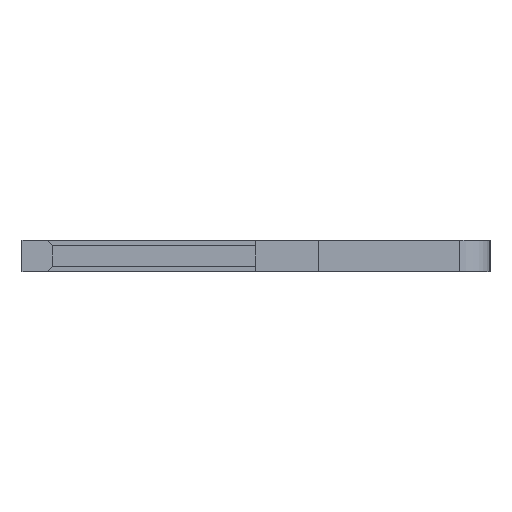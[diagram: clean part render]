
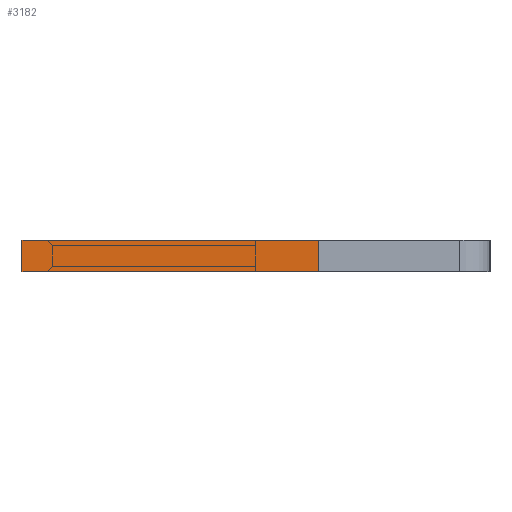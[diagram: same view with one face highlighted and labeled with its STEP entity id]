
A CAD part, left-side view. The second image highlights one B-rep face of the part: STEP entity #3182.
In plain terms, the highlighted face is planar.
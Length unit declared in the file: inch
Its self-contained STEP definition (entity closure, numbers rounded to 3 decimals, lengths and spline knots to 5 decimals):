
#20 = LINE ( 'NONE', #1479, #3089 ) ;
#89 = ORIENTED_EDGE ( 'NONE', *, *, #2340, .T. ) ;
#145 = VERTEX_POINT ( 'NONE', #1949 ) ;
#252 = CARTESIAN_POINT ( 'NONE',  ( 0.01, 0.15, -0.04 ) ) ;
#434 = VECTOR ( 'NONE', #2036, 39.37008 ) ;
#546 = ORIENTED_EDGE ( 'NONE', *, *, #952, .F. ) ;
#728 = CARTESIAN_POINT ( 'NONE',  ( 0.01, -0.04, -0.04 ) ) ;
#780 = DIRECTION ( 'NONE',  ( 0., 1., 0. ) ) ;
#808 = CARTESIAN_POINT ( 'NONE',  ( 0.01, 0.15, -0.04 ) ) ;
#821 = PLANE ( 'NONE',  #4189 ) ;
#865 = EDGE_CURVE ( 'NONE', #3036, #145, #2927, .T. ) ;
#876 = ORIENTED_EDGE ( 'NONE', *, *, #865, .F. ) ;
#952 = EDGE_CURVE ( 'NONE', #4220, #3036, #3999, .T. ) ;
#1039 = ORIENTED_EDGE ( 'NONE', *, *, #2224, .T. ) ;
#1185 = CARTESIAN_POINT ( 'NONE',  ( 0.01, 0.15, -0.04 ) ) ;
#1450 = FACE_OUTER_BOUND ( 'NONE', #3519, .T. ) ;
#1479 = CARTESIAN_POINT ( 'NONE',  ( -0.01, 0.15, -0.04 ) ) ;
#1821 = CARTESIAN_POINT ( 'NONE',  ( -0.01, -0.04, -0.04 ) ) ;
#1866 = DIRECTION ( 'NONE',  ( 0., 0., 1. ) ) ;
#1949 = CARTESIAN_POINT ( 'NONE',  ( -0.01, 0.15, -0.04 ) ) ;
#2036 = DIRECTION ( 'NONE',  ( 0., 1., 0. ) ) ;
#2163 = VERTEX_POINT ( 'NONE', #1821 ) ;
#2224 = EDGE_CURVE ( 'NONE', #2163, #145, #20, .T. ) ;
#2340 = EDGE_CURVE ( 'NONE', #4220, #2163, #2808, .T. ) ;
#2715 = DIRECTION ( 'NONE',  ( -1., 0., 0. ) ) ;
#2808 = LINE ( 'NONE', #728, #3617 ) ;
#2920 = DIRECTION ( 'NONE',  ( 1., 0., 0. ) ) ;
#2927 = LINE ( 'NONE', #252, #3402 ) ;
#3036 = VERTEX_POINT ( 'NONE', #808 ) ;
#3089 = VECTOR ( 'NONE', #780, 39.37008 ) ;
#3182 = ADVANCED_FACE ( 'NONE', ( #1450 ), #821, .F. ) ;
#3402 = VECTOR ( 'NONE', #2715, 39.37008 ) ;
#3484 = DIRECTION ( 'NONE',  ( -1., 0., 0. ) ) ;
#3519 = EDGE_LOOP ( 'NONE', ( #1039, #876, #546, #89 ) ) ;
#3617 = VECTOR ( 'NONE', #3484, 39.37008 ) ;
#3921 = CARTESIAN_POINT ( 'NONE',  ( 0.01, -0.04, -0.04 ) ) ;
#3999 = LINE ( 'NONE', #4105, #434 ) ;
#4105 = CARTESIAN_POINT ( 'NONE',  ( 0.01, 0.15, -0.04 ) ) ;
#4189 = AXIS2_PLACEMENT_3D ( 'NONE', #1185, #1866, #2920 ) ;
#4220 = VERTEX_POINT ( 'NONE', #3921 ) ;
